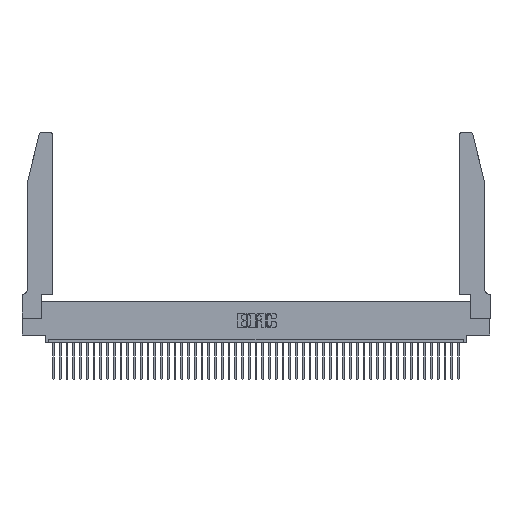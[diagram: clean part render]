
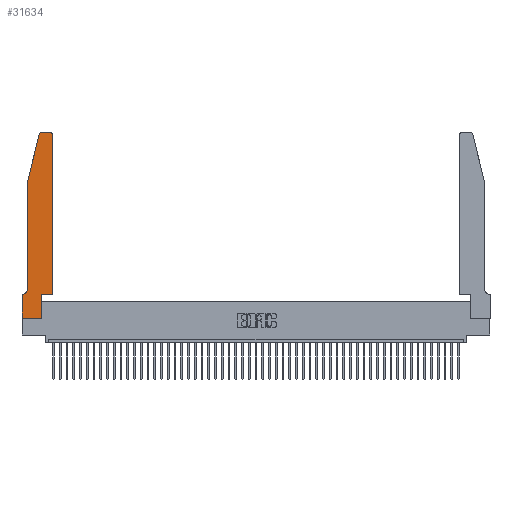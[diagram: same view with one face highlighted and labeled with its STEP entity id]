
A CAD part, top view. The second image highlights one B-rep face of the part: STEP entity #31634.
In plain terms, the highlighted planar face has unit normal (0, 0, 1).
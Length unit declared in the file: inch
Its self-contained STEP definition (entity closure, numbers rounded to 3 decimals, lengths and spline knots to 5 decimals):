
#238 = CARTESIAN_POINT ( 'NONE',  ( 0.0055, 0.42, 0.37 ) ) ;
#303 = ORIENTED_EDGE ( 'NONE', *, *, #11470, .T. ) ;
#325 = VERTEX_POINT ( 'NONE', #14595 ) ;
#521 = DIRECTION ( 'NONE',  ( 1., 0., 0. ) ) ;
#593 = ORIENTED_EDGE ( 'NONE', *, *, #18988, .T. ) ;
#1113 = CARTESIAN_POINT ( 'NONE',  ( 0., 0., 0.37 ) ) ;
#1136 = EDGE_CURVE ( 'NONE', #13804, #11040, #37811, .T. ) ;
#1244 = CARTESIAN_POINT ( 'NONE',  ( 0.4505, 0.35, 0.37 ) ) ;
#1935 = VECTOR ( 'NONE', #32868, 39.37008 ) ;
#2501 = CARTESIAN_POINT ( 'NONE',  ( 0.2865, 0.35, 0.37 ) ) ;
#3221 = LINE ( 'NONE', #44127, #41647 ) ;
#3491 = LINE ( 'NONE', #1113, #32037 ) ;
#4702 = CARTESIAN_POINT ( 'NONE',  ( 0.0755, 2., 0.37 ) ) ;
#4764 = CARTESIAN_POINT ( 'NONE',  ( 0.4505, 2.72, 0.37 ) ) ;
#4840 = DIRECTION ( 'NONE',  ( 0., -1., 0. ) ) ;
#7585 = LINE ( 'NONE', #27567, #11651 ) ;
#7605 = EDGE_CURVE ( 'NONE', #39792, #38533, #7585, .T. ) ;
#10577 = LINE ( 'NONE', #15581, #22779 ) ;
#11006 = LINE ( 'NONE', #13586, #26698 ) ;
#11040 = VERTEX_POINT ( 'NONE', #44642 ) ;
#11317 = CIRCLE ( 'NONE', #11689, 0.07 ) ;
#11408 = LINE ( 'NONE', #26793, #40046 ) ;
#11470 = EDGE_CURVE ( 'NONE', #325, #18205, #3491, .T. ) ;
#11584 = ORIENTED_EDGE ( 'NONE', *, *, #23826, .T. ) ;
#11651 = VECTOR ( 'NONE', #45711, 39.37008 ) ;
#11689 = AXIS2_PLACEMENT_3D ( 'NONE', #238, #37398, #26253 ) ;
#12349 = FACE_OUTER_BOUND ( 'NONE', #22512, .T. ) ;
#13150 = CARTESIAN_POINT ( 'NONE',  ( 0., 0.35, 0.37 ) ) ;
#13586 = CARTESIAN_POINT ( 'NONE',  ( 0.4505, 0.35, 0.37 ) ) ;
#13784 = DIRECTION ( 'NONE',  ( 0., 0., 1. ) ) ;
#13804 = VERTEX_POINT ( 'NONE', #21842 ) ;
#14096 = CARTESIAN_POINT ( 'NONE',  ( 0.2865, 0.35, 0.37 ) ) ;
#14595 = CARTESIAN_POINT ( 'NONE',  ( 0., 0., 0.37 ) ) ;
#15325 = LINE ( 'NONE', #14096, #1935 ) ;
#15581 = CARTESIAN_POINT ( 'NONE',  ( 0.2605, 2.75, 0.37 ) ) ;
#15676 = DIRECTION ( 'NONE',  ( 0., 0., 1. ) ) ;
#16553 = VECTOR ( 'NONE', #45290, 39.37008 ) ;
#17915 = CARTESIAN_POINT ( 'NONE',  ( 0.4205, 2.75, 0.37 ) ) ;
#18205 = VERTEX_POINT ( 'NONE', #42531 ) ;
#18401 = VERTEX_POINT ( 'NONE', #40857 ) ;
#18988 = EDGE_CURVE ( 'NONE', #47305, #325, #3221, .T. ) ;
#19007 = DIRECTION ( 'NONE',  ( -1., 0., 0. ) ) ;
#19587 = VERTEX_POINT ( 'NONE', #2501 ) ;
#19597 = VERTEX_POINT ( 'NONE', #22829 ) ;
#20001 = AXIS2_PLACEMENT_3D ( 'NONE', #28765, #13784, #43963 ) ;
#21842 = CARTESIAN_POINT ( 'NONE',  ( 0.284, 2.75, 0.37 ) ) ;
#22512 = EDGE_LOOP ( 'NONE', ( #34589, #47295, #46047, #32374, #36203, #23742, #593, #303, #30833, #11584, #29506, #40881 ) ) ;
#22664 = CARTESIAN_POINT ( 'NONE',  ( 0., 0.35, 0.37 ) ) ;
#22779 = VECTOR ( 'NONE', #19007, 39.37008 ) ;
#22829 = CARTESIAN_POINT ( 'NONE',  ( 0.0755, 2., 0.37 ) ) ;
#23742 = ORIENTED_EDGE ( 'NONE', *, *, #30798, .T. ) ;
#23826 = EDGE_CURVE ( 'NONE', #19587, #39792, #11006, .T. ) ;
#24343 = EDGE_CURVE ( 'NONE', #38533, #33503, #31379, .T. ) ;
#26253 = DIRECTION ( 'NONE',  ( -1., 0., 0. ) ) ;
#26423 = LINE ( 'NONE', #45119, #16553 ) ;
#26677 = EDGE_CURVE ( 'NONE', #11040, #19597, #46385, .T. ) ;
#26698 = VECTOR ( 'NONE', #47344, 39.37008 ) ;
#26793 = CARTESIAN_POINT ( 'NONE',  ( 0.0755, 2., 0.37 ) ) ;
#26863 = VERTEX_POINT ( 'NONE', #40833 ) ;
#27208 = CARTESIAN_POINT ( 'NONE',  ( 0.4205, 2.72, 0.37 ) ) ;
#27567 = CARTESIAN_POINT ( 'NONE',  ( 0.4505, 0.35, 0.37 ) ) ;
#28765 = CARTESIAN_POINT ( 'NONE',  ( 0.284, 2.72, 0.37 ) ) ;
#29506 = ORIENTED_EDGE ( 'NONE', *, *, #7605, .T. ) ;
#30798 = EDGE_CURVE ( 'NONE', #26863, #47305, #26423, .T. ) ;
#30810 = EDGE_CURVE ( 'NONE', #18401, #26863, #11317, .T. ) ;
#30833 = ORIENTED_EDGE ( 'NONE', *, *, #45572, .T. ) ;
#30891 = AXIS2_PLACEMENT_3D ( 'NONE', #27208, #38525, #38688 ) ;
#31189 = VECTOR ( 'NONE', #35367, 39.37008 ) ;
#31379 = CIRCLE ( 'NONE', #30891, 0.03 ) ;
#31634 = ADVANCED_FACE ( 'NONE', ( #12349 ), #45044, .T. ) ;
#32037 = VECTOR ( 'NONE', #38134, 39.37008 ) ;
#32374 = ORIENTED_EDGE ( 'NONE', *, *, #39892, .T. ) ;
#32868 = DIRECTION ( 'NONE',  ( 0., 1., 0. ) ) ;
#33026 = AXIS2_PLACEMENT_3D ( 'NONE', #22664, #15676, #521 ) ;
#33503 = VERTEX_POINT ( 'NONE', #17915 ) ;
#34589 = ORIENTED_EDGE ( 'NONE', *, *, #36876, .T. ) ;
#35367 = DIRECTION ( 'NONE',  ( -0.239, -0.971, 0. ) ) ;
#36203 = ORIENTED_EDGE ( 'NONE', *, *, #30810, .T. ) ;
#36876 = EDGE_CURVE ( 'NONE', #33503, #13804, #10577, .T. ) ;
#37398 = DIRECTION ( 'NONE',  ( 0., 0., -1. ) ) ;
#37811 = CIRCLE ( 'NONE', #20001, 0.03 ) ;
#37872 = DIRECTION ( 'NONE',  ( 0., -1., 0. ) ) ;
#38134 = DIRECTION ( 'NONE',  ( 1., 0., 0. ) ) ;
#38525 = DIRECTION ( 'NONE',  ( 0., 0., 1. ) ) ;
#38533 = VERTEX_POINT ( 'NONE', #4764 ) ;
#38688 = DIRECTION ( 'NONE',  ( 1., 0., 0. ) ) ;
#39792 = VERTEX_POINT ( 'NONE', #1244 ) ;
#39892 = EDGE_CURVE ( 'NONE', #19597, #18401, #11408, .T. ) ;
#40046 = VECTOR ( 'NONE', #4840, 39.37008 ) ;
#40833 = CARTESIAN_POINT ( 'NONE',  ( 0.0055, 0.35, 0.37 ) ) ;
#40857 = CARTESIAN_POINT ( 'NONE',  ( 0.0755, 0.42, 0.37 ) ) ;
#40881 = ORIENTED_EDGE ( 'NONE', *, *, #24343, .T. ) ;
#41647 = VECTOR ( 'NONE', #37872, 39.37008 ) ;
#42531 = CARTESIAN_POINT ( 'NONE',  ( 0.2865, 0., 0.37 ) ) ;
#43963 = DIRECTION ( 'NONE',  ( 1., 0., 0. ) ) ;
#44127 = CARTESIAN_POINT ( 'NONE',  ( 0., 0., 0.37 ) ) ;
#44642 = CARTESIAN_POINT ( 'NONE',  ( 0.25487, 2.72718, 0.37 ) ) ;
#45044 = PLANE ( 'NONE',  #33026 ) ;
#45119 = CARTESIAN_POINT ( 'NONE',  ( 0.0755, 0.35, 0.37 ) ) ;
#45290 = DIRECTION ( 'NONE',  ( -1., 0., 0. ) ) ;
#45572 = EDGE_CURVE ( 'NONE', #18205, #19587, #15325, .T. ) ;
#45711 = DIRECTION ( 'NONE',  ( 0., 1., 0. ) ) ;
#46047 = ORIENTED_EDGE ( 'NONE', *, *, #26677, .T. ) ;
#46385 = LINE ( 'NONE', #4702, #31189 ) ;
#47295 = ORIENTED_EDGE ( 'NONE', *, *, #1136, .T. ) ;
#47305 = VERTEX_POINT ( 'NONE', #13150 ) ;
#47344 = DIRECTION ( 'NONE',  ( 1., 0., 0. ) ) ;
